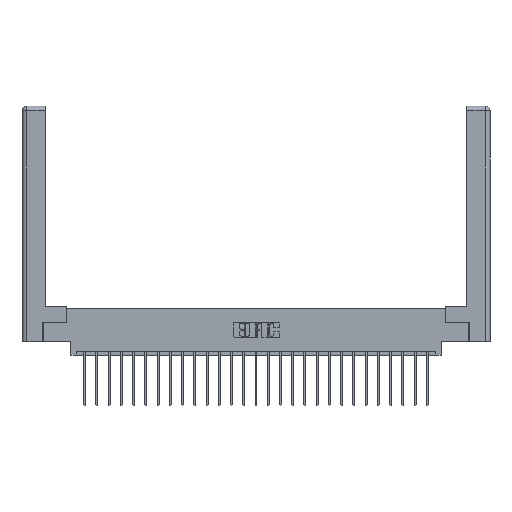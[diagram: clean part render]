
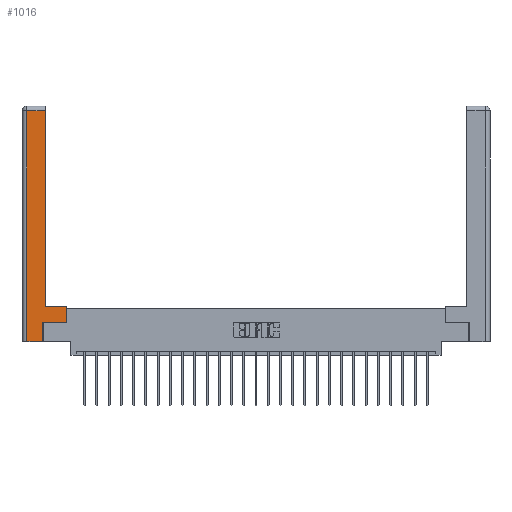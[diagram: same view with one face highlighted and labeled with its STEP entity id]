
A CAD part, top view. The second image highlights one B-rep face of the part: STEP entity #1016.
In plain terms, the highlighted planar face has unit normal (0, 0, 1).
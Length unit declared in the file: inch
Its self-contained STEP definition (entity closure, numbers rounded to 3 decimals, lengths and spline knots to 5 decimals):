
#47 = DIRECTION ( 'NONE',  ( -1., 0., 0. ) ) ;
#385 = VECTOR ( 'NONE', #23033, 39.37008 ) ;
#585 = EDGE_CURVE ( 'NONE', #22506, #18378, #4945, .T. ) ;
#662 = CARTESIAN_POINT ( 'NONE',  ( 0.565, 0.245, 0. ) ) ;
#698 = LINE ( 'NONE', #14710, #18291 ) ;
#1016 = ADVANCED_FACE ( 'NONE', ( #5890 ), #4314, .F. ) ;
#1036 = LINE ( 'NONE', #12104, #385 ) ;
#1131 = CARTESIAN_POINT ( 'NONE',  ( 0.295, 0.45, 0. ) ) ;
#1203 = EDGE_CURVE ( 'NONE', #17222, #12818, #698, .T. ) ;
#1868 = CARTESIAN_POINT ( 'NONE',  ( 0.295, 3., 0. ) ) ;
#2377 = EDGE_CURVE ( 'NONE', #20837, #18022, #17448, .T. ) ;
#2609 = EDGE_CURVE ( 'NONE', #18378, #17222, #25226, .T. ) ;
#2625 = ORIENTED_EDGE ( 'NONE', *, *, #585, .T. ) ;
#3960 = VECTOR ( 'NONE', #6809, 39.37008 ) ;
#4240 = DIRECTION ( 'NONE',  ( 1., 0., 0. ) ) ;
#4314 = PLANE ( 'NONE',  #8189 ) ;
#4703 = VECTOR ( 'NONE', #16289, 39.37008 ) ;
#4945 = LINE ( 'NONE', #10503, #12124 ) ;
#5890 = FACE_OUTER_BOUND ( 'NONE', #18876, .T. ) ;
#6651 = DIRECTION ( 'NONE',  ( -1., 0., 0. ) ) ;
#6809 = DIRECTION ( 'NONE',  ( 0., 1., 0. ) ) ;
#6938 = LINE ( 'NONE', #15161, #16756 ) ;
#7120 = DIRECTION ( 'NONE',  ( 0., -1., 0. ) ) ;
#7705 = CARTESIAN_POINT ( 'NONE',  ( 0.265, 0., 0. ) ) ;
#8189 = AXIS2_PLACEMENT_3D ( 'NONE', #8789, #10418, #16746 ) ;
#8257 = VERTEX_POINT ( 'NONE', #25596 ) ;
#8651 = EDGE_CURVE ( 'NONE', #8257, #24380, #6938, .T. ) ;
#8789 = CARTESIAN_POINT ( 'NONE',  ( 0., 0., 0. ) ) ;
#8847 = CARTESIAN_POINT ( 'NONE',  ( 0.565, 0.45, 0. ) ) ;
#8884 = CARTESIAN_POINT ( 'NONE',  ( 0.565, 0.45, 0. ) ) ;
#9322 = CARTESIAN_POINT ( 'NONE',  ( 0.265, 0.245, 0. ) ) ;
#9525 = LINE ( 'NONE', #8847, #3960 ) ;
#9702 = VECTOR ( 'NONE', #7120, 39.37008 ) ;
#10080 = CARTESIAN_POINT ( 'NONE',  ( 0.295, 2.94, 0. ) ) ;
#10418 = DIRECTION ( 'NONE',  ( 0., 0., -1. ) ) ;
#10503 = CARTESIAN_POINT ( 'NONE',  ( 0.295, 0.45, 0. ) ) ;
#10811 = CARTESIAN_POINT ( 'NONE',  ( 0.565, 0.245, 0. ) ) ;
#11157 = ORIENTED_EDGE ( 'NONE', *, *, #19657, .T. ) ;
#11555 = VECTOR ( 'NONE', #19836, 39.37008 ) ;
#12104 = CARTESIAN_POINT ( 'NONE',  ( 0.265, 0.245, 0. ) ) ;
#12124 = VECTOR ( 'NONE', #47, 39.37008 ) ;
#12818 = VERTEX_POINT ( 'NONE', #18054 ) ;
#14710 = CARTESIAN_POINT ( 'NONE',  ( 0.0615, 2.94, 0. ) ) ;
#15161 = CARTESIAN_POINT ( 'NONE',  ( 0.265, 0., 0. ) ) ;
#15360 = ORIENTED_EDGE ( 'NONE', *, *, #16937, .T. ) ;
#15600 = ORIENTED_EDGE ( 'NONE', *, *, #1203, .T. ) ;
#16289 = DIRECTION ( 'NONE',  ( 0., 1., 0. ) ) ;
#16746 = DIRECTION ( 'NONE',  ( -1., 0., 0. ) ) ;
#16756 = VECTOR ( 'NONE', #4240, 39.37008 ) ;
#16824 = ORIENTED_EDGE ( 'NONE', *, *, #23793, .T. ) ;
#16937 = EDGE_CURVE ( 'NONE', #24380, #20837, #1036, .T. ) ;
#17222 = VERTEX_POINT ( 'NONE', #10080 ) ;
#17448 = LINE ( 'NONE', #10811, #11555 ) ;
#17576 = ORIENTED_EDGE ( 'NONE', *, *, #2609, .T. ) ;
#18022 = VERTEX_POINT ( 'NONE', #662 ) ;
#18054 = CARTESIAN_POINT ( 'NONE',  ( 0.0615, 2.94, 0. ) ) ;
#18291 = VECTOR ( 'NONE', #6651, 39.37008 ) ;
#18378 = VERTEX_POINT ( 'NONE', #1131 ) ;
#18876 = EDGE_LOOP ( 'NONE', ( #17576, #15600, #11157, #19054, #15360, #20538, #16824, #2625 ) ) ;
#19054 = ORIENTED_EDGE ( 'NONE', *, *, #8651, .T. ) ;
#19470 = LINE ( 'NONE', #25787, #9702 ) ;
#19657 = EDGE_CURVE ( 'NONE', #12818, #8257, #19470, .T. ) ;
#19836 = DIRECTION ( 'NONE',  ( 1., 0., 0. ) ) ;
#20538 = ORIENTED_EDGE ( 'NONE', *, *, #2377, .T. ) ;
#20837 = VERTEX_POINT ( 'NONE', #9322 ) ;
#22506 = VERTEX_POINT ( 'NONE', #8884 ) ;
#23033 = DIRECTION ( 'NONE',  ( 0., 1., 0. ) ) ;
#23793 = EDGE_CURVE ( 'NONE', #18022, #22506, #9525, .T. ) ;
#24380 = VERTEX_POINT ( 'NONE', #7705 ) ;
#25226 = LINE ( 'NONE', #1868, #4703 ) ;
#25596 = CARTESIAN_POINT ( 'NONE',  ( 0.0615, 0., 0. ) ) ;
#25787 = CARTESIAN_POINT ( 'NONE',  ( 0.0615, 0., 0. ) ) ;
